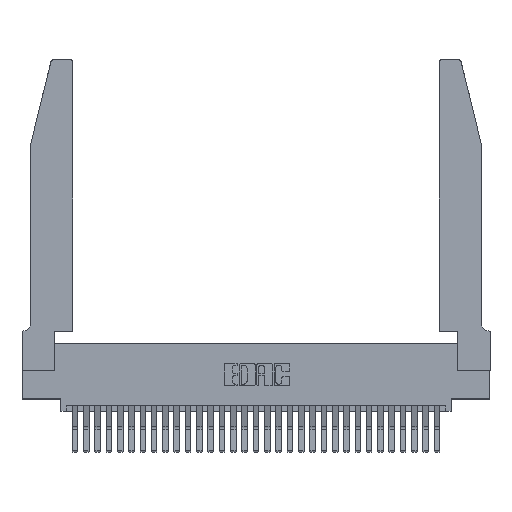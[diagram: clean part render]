
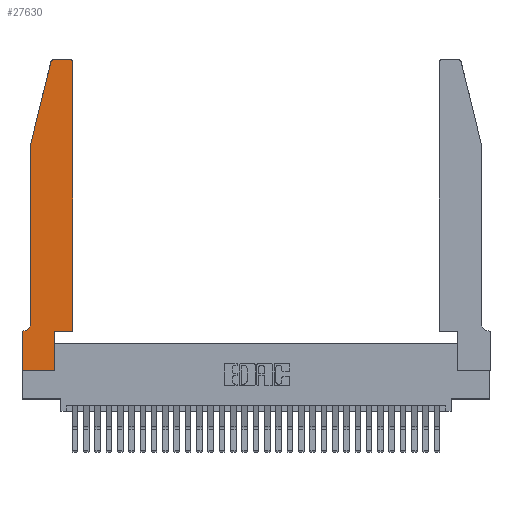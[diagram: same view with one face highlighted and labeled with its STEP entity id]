
A CAD part, top view. The second image highlights one B-rep face of the part: STEP entity #27630.
In plain terms, the highlighted planar face has unit normal (0, 0, 1).
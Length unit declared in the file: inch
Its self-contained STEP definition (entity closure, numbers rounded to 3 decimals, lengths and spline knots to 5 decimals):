
#140 = ORIENTED_EDGE ( 'NONE', *, *, #24114, .T. ) ;
#215 = EDGE_CURVE ( 'NONE', #25148, #13189, #20696, .T. ) ;
#678 = CARTESIAN_POINT ( 'NONE',  ( 0.2605, 2.75, 0.37 ) ) ;
#828 = CARTESIAN_POINT ( 'NONE',  ( 0., 0., 0.37 ) ) ;
#846 = CARTESIAN_POINT ( 'NONE',  ( 0.4505, 0.35, 0.37 ) ) ;
#1458 = LINE ( 'NONE', #828, #15432 ) ;
#1598 = EDGE_CURVE ( 'NONE', #14248, #20242, #2719, .T. ) ;
#1988 = DIRECTION ( 'NONE',  ( 1., 0., 0. ) ) ;
#2178 = AXIS2_PLACEMENT_3D ( 'NONE', #24229, #8927, #14041 ) ;
#2352 = CARTESIAN_POINT ( 'NONE',  ( 0.4205, 2.72, 0.37 ) ) ;
#2719 = LINE ( 'NONE', #24053, #26747 ) ;
#2807 = ORIENTED_EDGE ( 'NONE', *, *, #23279, .T. ) ;
#2840 = VECTOR ( 'NONE', #21369, 39.37008 ) ;
#2930 = VECTOR ( 'NONE', #12785, 39.37008 ) ;
#3187 = VERTEX_POINT ( 'NONE', #9869 ) ;
#3976 = CARTESIAN_POINT ( 'NONE',  ( 0.284, 2.75, 0.37 ) ) ;
#4018 = EDGE_CURVE ( 'NONE', #20242, #3187, #18890, .T. ) ;
#4252 = DIRECTION ( 'NONE',  ( 0., 0., 1. ) ) ;
#4371 = CARTESIAN_POINT ( 'NONE',  ( 0., 0.35, 0.37 ) ) ;
#5901 = CARTESIAN_POINT ( 'NONE',  ( 0.0755, 2., 0.37 ) ) ;
#6152 = LINE ( 'NONE', #6201, #31746 ) ;
#6201 = CARTESIAN_POINT ( 'NONE',  ( 0.2865, 0.35, 0.37 ) ) ;
#6848 = CIRCLE ( 'NONE', #2178, 0.03 ) ;
#8179 = DIRECTION ( 'NONE',  ( 1., 0., 0. ) ) ;
#8481 = DIRECTION ( 'NONE',  ( 0., 0., -1. ) ) ;
#8777 = CARTESIAN_POINT ( 'NONE',  ( 0.0055, 0.42, 0.37 ) ) ;
#8871 = CARTESIAN_POINT ( 'NONE',  ( 0.4505, 0.35, 0.37 ) ) ;
#8927 = DIRECTION ( 'NONE',  ( 0., 0., 1. ) ) ;
#9869 = CARTESIAN_POINT ( 'NONE',  ( 0.0755, 0.42, 0.37 ) ) ;
#10029 = ORIENTED_EDGE ( 'NONE', *, *, #29023, .T. ) ;
#10278 = ORIENTED_EDGE ( 'NONE', *, *, #1598, .T. ) ;
#10491 = EDGE_CURVE ( 'NONE', #12664, #17157, #6152, .T. ) ;
#10672 = DIRECTION ( 'NONE',  ( -1., 0., 0. ) ) ;
#10748 = AXIS2_PLACEMENT_3D ( 'NONE', #4371, #4252, #1988 ) ;
#11171 = ORIENTED_EDGE ( 'NONE', *, *, #20559, .T. ) ;
#11231 = EDGE_CURVE ( 'NONE', #21354, #25148, #23580, .T. ) ;
#11237 = CARTESIAN_POINT ( 'NONE',  ( 0., 0., 0.37 ) ) ;
#11514 = ORIENTED_EDGE ( 'NONE', *, *, #11231, .T. ) ;
#11702 = AXIS2_PLACEMENT_3D ( 'NONE', #8777, #8481, #10672 ) ;
#12111 = CARTESIAN_POINT ( 'NONE',  ( 0.0755, 0.35, 0.37 ) ) ;
#12319 = CARTESIAN_POINT ( 'NONE',  ( 0.4505, 0.35, 0.37 ) ) ;
#12664 = VERTEX_POINT ( 'NONE', #22137 ) ;
#12704 = VECTOR ( 'NONE', #27235, 39.37008 ) ;
#12785 = DIRECTION ( 'NONE',  ( 0., -1., 0. ) ) ;
#12973 = EDGE_CURVE ( 'NONE', #3187, #20529, #29316, .T. ) ;
#13189 = VERTEX_POINT ( 'NONE', #30366 ) ;
#13858 = CARTESIAN_POINT ( 'NONE',  ( 0.0055, 0.35, 0.37 ) ) ;
#14041 = DIRECTION ( 'NONE',  ( 1., 0., 0. ) ) ;
#14248 = VERTEX_POINT ( 'NONE', #14499 ) ;
#14499 = CARTESIAN_POINT ( 'NONE',  ( 0.25487, 2.72718, 0.37 ) ) ;
#14875 = ORIENTED_EDGE ( 'NONE', *, *, #4018, .T. ) ;
#15432 = VECTOR ( 'NONE', #8179, 39.37008 ) ;
#16132 = CARTESIAN_POINT ( 'NONE',  ( 0., 0.35, 0.37 ) ) ;
#16880 = AXIS2_PLACEMENT_3D ( 'NONE', #2352, #22310, #17013 ) ;
#16889 = VERTEX_POINT ( 'NONE', #11237 ) ;
#17013 = DIRECTION ( 'NONE',  ( 1., 0., 0. ) ) ;
#17157 = VERTEX_POINT ( 'NONE', #29780 ) ;
#17885 = EDGE_CURVE ( 'NONE', #13189, #20585, #24083, .T. ) ;
#18666 = DIRECTION ( 'NONE',  ( 1., 0., 0. ) ) ;
#18890 = LINE ( 'NONE', #27905, #2930 ) ;
#19203 = CARTESIAN_POINT ( 'NONE',  ( 0.4505, 2.72, 0.37 ) ) ;
#19256 = ORIENTED_EDGE ( 'NONE', *, *, #10491, .T. ) ;
#20242 = VERTEX_POINT ( 'NONE', #5901 ) ;
#20348 = LINE ( 'NONE', #31162, #2840 ) ;
#20479 = DIRECTION ( 'NONE',  ( -1., 0., 0. ) ) ;
#20487 = LINE ( 'NONE', #12111, #12704 ) ;
#20529 = VERTEX_POINT ( 'NONE', #13858 ) ;
#20559 = EDGE_CURVE ( 'NONE', #23912, #16889, #20348, .T. ) ;
#20585 = VERTEX_POINT ( 'NONE', #3976 ) ;
#20696 = CIRCLE ( 'NONE', #16880, 0.03 ) ;
#21354 = VERTEX_POINT ( 'NONE', #12319 ) ;
#21369 = DIRECTION ( 'NONE',  ( 0., -1., 0. ) ) ;
#22137 = CARTESIAN_POINT ( 'NONE',  ( 0.2865, 0., 0.37 ) ) ;
#22310 = DIRECTION ( 'NONE',  ( 0., 0., 1. ) ) ;
#22905 = ORIENTED_EDGE ( 'NONE', *, *, #215, .T. ) ;
#23279 = EDGE_CURVE ( 'NONE', #17157, #21354, #27096, .T. ) ;
#23308 = VECTOR ( 'NONE', #20479, 39.37008 ) ;
#23580 = LINE ( 'NONE', #8871, #25860 ) ;
#23912 = VERTEX_POINT ( 'NONE', #16132 ) ;
#24053 = CARTESIAN_POINT ( 'NONE',  ( 0.0755, 2., 0.37 ) ) ;
#24083 = LINE ( 'NONE', #678, #23308 ) ;
#24114 = EDGE_CURVE ( 'NONE', #20585, #14248, #6848, .T. ) ;
#24229 = CARTESIAN_POINT ( 'NONE',  ( 0.284, 2.72, 0.37 ) ) ;
#24836 = ORIENTED_EDGE ( 'NONE', *, *, #28649, .T. ) ;
#25148 = VERTEX_POINT ( 'NONE', #19203 ) ;
#25860 = VECTOR ( 'NONE', #31184, 39.37008 ) ;
#26747 = VECTOR ( 'NONE', #31590, 39.37008 ) ;
#26885 = PLANE ( 'NONE',  #10748 ) ;
#27096 = LINE ( 'NONE', #846, #31355 ) ;
#27235 = DIRECTION ( 'NONE',  ( -1., 0., 0. ) ) ;
#27630 = ADVANCED_FACE ( 'NONE', ( #31767 ), #26885, .T. ) ;
#27905 = CARTESIAN_POINT ( 'NONE',  ( 0.0755, 2., 0.37 ) ) ;
#28523 = DIRECTION ( 'NONE',  ( 0., 1., 0. ) ) ;
#28649 = EDGE_CURVE ( 'NONE', #16889, #12664, #1458, .T. ) ;
#29023 = EDGE_CURVE ( 'NONE', #20529, #23912, #20487, .T. ) ;
#29316 = CIRCLE ( 'NONE', #11702, 0.07 ) ;
#29780 = CARTESIAN_POINT ( 'NONE',  ( 0.2865, 0.35, 0.37 ) ) ;
#30059 = ORIENTED_EDGE ( 'NONE', *, *, #12973, .T. ) ;
#30366 = CARTESIAN_POINT ( 'NONE',  ( 0.4205, 2.75, 0.37 ) ) ;
#31162 = CARTESIAN_POINT ( 'NONE',  ( 0., 0., 0.37 ) ) ;
#31184 = DIRECTION ( 'NONE',  ( 0., 1., 0. ) ) ;
#31197 = EDGE_LOOP ( 'NONE', ( #31420, #140, #10278, #14875, #30059, #10029, #11171, #24836, #19256, #2807, #11514, #22905 ) ) ;
#31355 = VECTOR ( 'NONE', #18666, 39.37008 ) ;
#31420 = ORIENTED_EDGE ( 'NONE', *, *, #17885, .T. ) ;
#31590 = DIRECTION ( 'NONE',  ( -0.239, -0.971, 0. ) ) ;
#31746 = VECTOR ( 'NONE', #28523, 39.37008 ) ;
#31767 = FACE_OUTER_BOUND ( 'NONE', #31197, .T. ) ;
